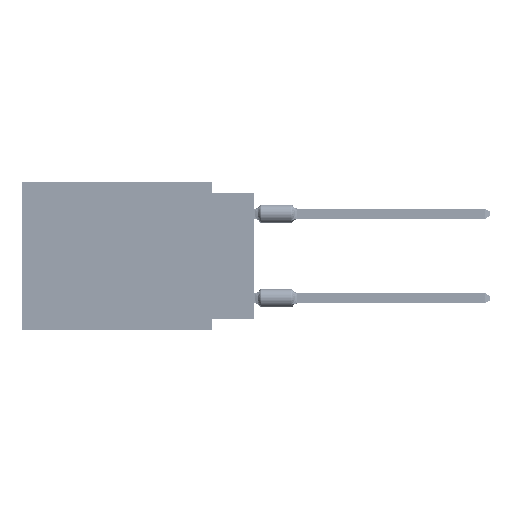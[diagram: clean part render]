
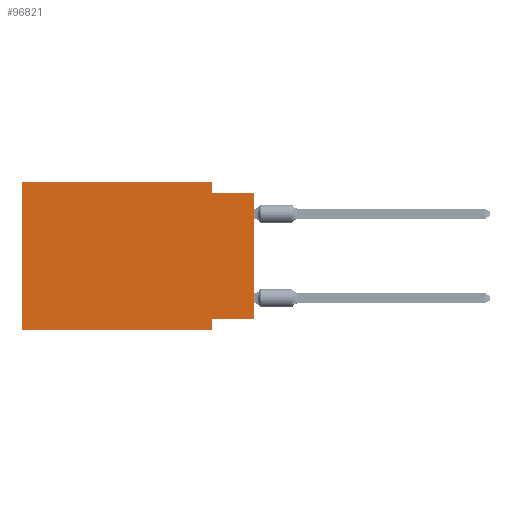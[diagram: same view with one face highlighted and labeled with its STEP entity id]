
A CAD part, left-side view. The second image highlights one B-rep face of the part: STEP entity #96821.
In plain terms, the highlighted planar face has unit normal (-1, 0, 0).
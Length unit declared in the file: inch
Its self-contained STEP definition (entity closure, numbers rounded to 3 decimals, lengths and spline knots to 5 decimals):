
#879 = VECTOR ( 'NONE', #8847, 39.37008 ) ;
#1091 = VERTEX_POINT ( 'NONE', #24054 ) ;
#3681 = VECTOR ( 'NONE', #19484, 39.37008 ) ;
#4331 = LINE ( 'NONE', #107861, #94136 ) ;
#4812 = CARTESIAN_POINT ( 'NONE',  ( 0., 0.55, 0. ) ) ;
#5955 = DIRECTION ( 'NONE',  ( 0., 0., -1. ) ) ;
#7343 = DIRECTION ( 'NONE',  ( 0., 0., 1. ) ) ;
#7450 = EDGE_LOOP ( 'NONE', ( #55425, #37151, #16152, #70927, #74976, #71023, #34530, #76203 ) ) ;
#8847 = DIRECTION ( 'NONE',  ( 0., 0., 1. ) ) ;
#12344 = CARTESIAN_POINT ( 'NONE',  ( 0., 0., -0.325 ) ) ;
#14363 = VERTEX_POINT ( 'NONE', #112095 ) ;
#16016 = VERTEX_POINT ( 'NONE', #40355 ) ;
#16152 = ORIENTED_EDGE ( 'NONE', *, *, #23868, .F. ) ;
#18073 = LINE ( 'NONE', #45394, #24871 ) ;
#18649 = EDGE_CURVE ( 'NONE', #111051, #57498, #54738, .T. ) ;
#19484 = DIRECTION ( 'NONE',  ( 0., 1., 0. ) ) ;
#22514 = CARTESIAN_POINT ( 'NONE',  ( 0., 0.1, -0.025 ) ) ;
#23868 = EDGE_CURVE ( 'NONE', #16016, #47912, #4331, .T. ) ;
#24054 = CARTESIAN_POINT ( 'NONE',  ( 0., 0.55, 0. ) ) ;
#24871 = VECTOR ( 'NONE', #96538, 39.37008 ) ;
#27459 = VERTEX_POINT ( 'NONE', #88658 ) ;
#29118 = VERTEX_POINT ( 'NONE', #100427 ) ;
#31154 = EDGE_CURVE ( 'NONE', #1091, #16016, #88375, .T. ) ;
#32408 = LINE ( 'NONE', #33554, #84025 ) ;
#33554 = CARTESIAN_POINT ( 'NONE',  ( 0., 0.55, 0. ) ) ;
#34530 = ORIENTED_EDGE ( 'NONE', *, *, #103441, .F. ) ;
#36676 = CARTESIAN_POINT ( 'NONE',  ( 0., 0.55, 0. ) ) ;
#36906 = AXIS2_PLACEMENT_3D ( 'NONE', #4812, #83836, #5955 ) ;
#37151 = ORIENTED_EDGE ( 'NONE', *, *, #83782, .F. ) ;
#37610 = DIRECTION ( 'NONE',  ( 0., 0., -1. ) ) ;
#40355 = CARTESIAN_POINT ( 'NONE',  ( 0., 0.1, 0. ) ) ;
#43904 = CARTESIAN_POINT ( 'NONE',  ( 0., 0.1, -0.35 ) ) ;
#45394 = CARTESIAN_POINT ( 'NONE',  ( 0., 0.55, -0.35 ) ) ;
#47912 = VERTEX_POINT ( 'NONE', #22514 ) ;
#48069 = PLANE ( 'NONE',  #36906 ) ;
#49189 = FACE_OUTER_BOUND ( 'NONE', #7450, .T. ) ;
#49425 = EDGE_CURVE ( 'NONE', #29118, #14363, #18073, .T. ) ;
#52011 = CARTESIAN_POINT ( 'NONE',  ( 0., 0., -0.025 ) ) ;
#54738 = LINE ( 'NONE', #64369, #3681 ) ;
#55425 = ORIENTED_EDGE ( 'NONE', *, *, #101249, .T. ) ;
#56037 = CARTESIAN_POINT ( 'NONE',  ( 0., 0.1, -0.325 ) ) ;
#56983 = VECTOR ( 'NONE', #86659, 39.37008 ) ;
#57498 = VERTEX_POINT ( 'NONE', #56037 ) ;
#60609 = LINE ( 'NONE', #86744, #879 ) ;
#61481 = LINE ( 'NONE', #43904, #70279 ) ;
#64369 = CARTESIAN_POINT ( 'NONE',  ( 0., 0., -0.325 ) ) ;
#70279 = VECTOR ( 'NONE', #37610, 39.37008 ) ;
#70927 = ORIENTED_EDGE ( 'NONE', *, *, #31154, .F. ) ;
#71023 = ORIENTED_EDGE ( 'NONE', *, *, #49425, .T. ) ;
#73156 = DIRECTION ( 'NONE',  ( 0., 0., -1. ) ) ;
#74976 = ORIENTED_EDGE ( 'NONE', *, *, #82788, .F. ) ;
#76203 = ORIENTED_EDGE ( 'NONE', *, *, #18649, .F. ) ;
#82788 = EDGE_CURVE ( 'NONE', #29118, #1091, #32408, .T. ) ;
#83782 = EDGE_CURVE ( 'NONE', #47912, #27459, #96311, .T. ) ;
#83836 = DIRECTION ( 'NONE',  ( 1., 0., 0. ) ) ;
#84025 = VECTOR ( 'NONE', #7343, 39.37008 ) ;
#85685 = VECTOR ( 'NONE', #87238, 39.37008 ) ;
#86659 = DIRECTION ( 'NONE',  ( 0., -1., 0. ) ) ;
#86744 = CARTESIAN_POINT ( 'NONE',  ( 0., 0., 0. ) ) ;
#87238 = DIRECTION ( 'NONE',  ( 0., -1., 0. ) ) ;
#88375 = LINE ( 'NONE', #36676, #85685 ) ;
#88658 = CARTESIAN_POINT ( 'NONE',  ( 0., 0., -0.025 ) ) ;
#94136 = VECTOR ( 'NONE', #73156, 39.37008 ) ;
#96311 = LINE ( 'NONE', #52011, #56983 ) ;
#96538 = DIRECTION ( 'NONE',  ( 0., -1., 0. ) ) ;
#96821 = ADVANCED_FACE ( 'NONE', ( #49189 ), #48069, .F. ) ;
#100427 = CARTESIAN_POINT ( 'NONE',  ( 0., 0.55, -0.35 ) ) ;
#101249 = EDGE_CURVE ( 'NONE', #111051, #27459, #60609, .T. ) ;
#103441 = EDGE_CURVE ( 'NONE', #57498, #14363, #61481, .T. ) ;
#107861 = CARTESIAN_POINT ( 'NONE',  ( 0., 0.1, 0. ) ) ;
#111051 = VERTEX_POINT ( 'NONE', #12344 ) ;
#112095 = CARTESIAN_POINT ( 'NONE',  ( 0., 0.1, -0.35 ) ) ;
